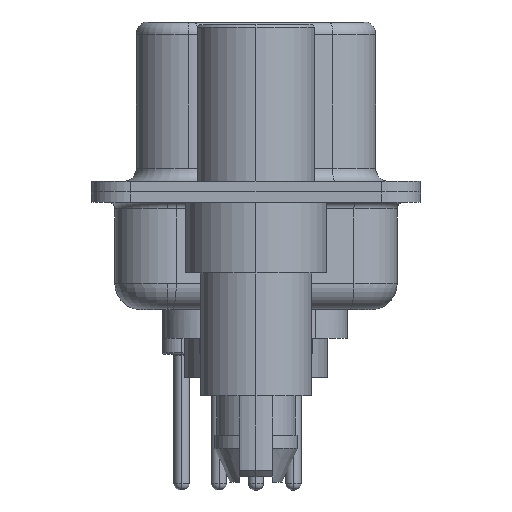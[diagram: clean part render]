
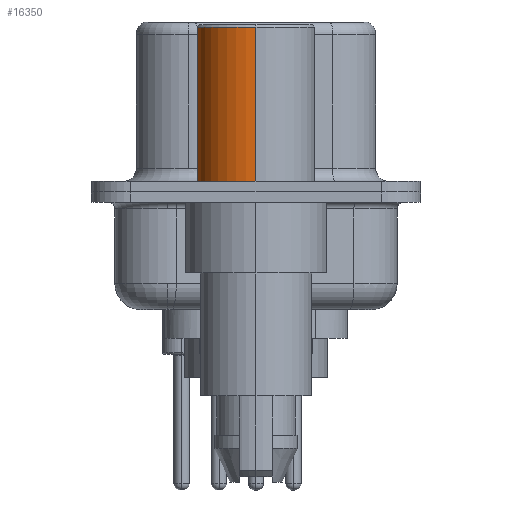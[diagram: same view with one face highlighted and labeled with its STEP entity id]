
A CAD part, left-side view. The second image highlights one B-rep face of the part: STEP entity #16350.
In plain terms, the highlighted cylindrical face has radius 2.25 mm (diameter 4.5 mm), a partial arc.
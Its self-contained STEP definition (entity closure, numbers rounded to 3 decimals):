
#516 = VECTOR ( 'NONE', #10205, 1000. ) ;
#1167 = DIRECTION ( 'NONE',  ( 0., 0., 1. ) ) ;
#1769 = CARTESIAN_POINT ( 'NONE',  ( 2.25, 0., 6.3 ) ) ;
#2417 = AXIS2_PLACEMENT_3D ( 'NONE', #14345, #17230, #9161 ) ;
#2759 = EDGE_CURVE ( 'NONE', #16794, #3697, #6850, .T. ) ;
#2976 = AXIS2_PLACEMENT_3D ( 'NONE', #20182, #13642, #4095 ) ;
#3151 = EDGE_CURVE ( 'NONE', #3697, #9076, #16503, .T. ) ;
#3216 = DIRECTION ( 'NONE',  ( 0., 0., 1. ) ) ;
#3697 = VERTEX_POINT ( 'NONE', #15672 ) ;
#3781 = VERTEX_POINT ( 'NONE', #1769 ) ;
#4095 = DIRECTION ( 'NONE',  ( 1., 0., 0. ) ) ;
#4564 = ORIENTED_EDGE ( 'NONE', *, *, #2759, .T. ) ;
#5987 = EDGE_CURVE ( 'NONE', #16794, #3781, #16403, .T. ) ;
#6291 = CARTESIAN_POINT ( 'NONE',  ( 2.25, 0., 0.581 ) ) ;
#6850 = CIRCLE ( 'NONE', #2976, 2.25 ) ;
#7597 = CARTESIAN_POINT ( 'NONE',  ( 2.25, 0., 0.4 ) ) ;
#7696 = CARTESIAN_POINT ( 'NONE',  ( -2.25, 0., 6.3 ) ) ;
#8253 = EDGE_LOOP ( 'NONE', ( #4564, #14078, #20956, #15946 ) ) ;
#8650 = CARTESIAN_POINT ( 'NONE',  ( -2.25, 0., 0.581 ) ) ;
#9076 = VERTEX_POINT ( 'NONE', #7696 ) ;
#9161 = DIRECTION ( 'NONE',  ( 1., 0., 0. ) ) ;
#9457 = CARTESIAN_POINT ( 'NONE',  ( 0., 0., 0.581 ) ) ;
#10205 = DIRECTION ( 'NONE',  ( 0., 0., 1. ) ) ;
#11065 = CYLINDRICAL_SURFACE ( 'NONE', #17365, 2.25 ) ;
#11125 = CIRCLE ( 'NONE', #2417, 2.25 ) ;
#13642 = DIRECTION ( 'NONE',  ( 0., 0., 1. ) ) ;
#14078 = ORIENTED_EDGE ( 'NONE', *, *, #3151, .T. ) ;
#14345 = CARTESIAN_POINT ( 'NONE',  ( 0., 0., 6.3 ) ) ;
#14807 = EDGE_CURVE ( 'NONE', #3781, #9076, #11125, .T. ) ;
#15672 = CARTESIAN_POINT ( 'NONE',  ( -2.25, 0., 0.4 ) ) ;
#15870 = VECTOR ( 'NONE', #3216, 1000. ) ;
#15946 = ORIENTED_EDGE ( 'NONE', *, *, #5987, .F. ) ;
#16350 = ADVANCED_FACE ( 'NONE', ( #20213 ), #11065, .T. ) ;
#16403 = LINE ( 'NONE', #6291, #15870 ) ;
#16503 = LINE ( 'NONE', #8650, #516 ) ;
#16794 = VERTEX_POINT ( 'NONE', #7597 ) ;
#17230 = DIRECTION ( 'NONE',  ( 0., 0., 1. ) ) ;
#17365 = AXIS2_PLACEMENT_3D ( 'NONE', #9457, #1167, #17527 ) ;
#17527 = DIRECTION ( 'NONE',  ( 1., 0., 0. ) ) ;
#20182 = CARTESIAN_POINT ( 'NONE',  ( 0., 0., 0.4 ) ) ;
#20213 = FACE_OUTER_BOUND ( 'NONE', #8253, .T. ) ;
#20956 = ORIENTED_EDGE ( 'NONE', *, *, #14807, .F. ) ;
